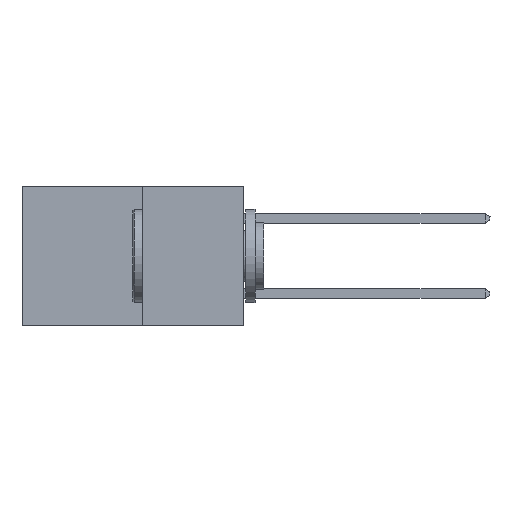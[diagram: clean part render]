
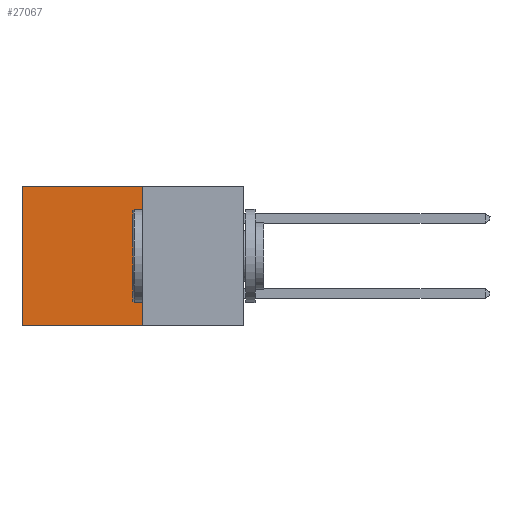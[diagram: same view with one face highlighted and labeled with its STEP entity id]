
A CAD part, left-side view. The second image highlights one B-rep face of the part: STEP entity #27067.
In plain terms, the highlighted planar face has unit normal (-1, 0, 0).
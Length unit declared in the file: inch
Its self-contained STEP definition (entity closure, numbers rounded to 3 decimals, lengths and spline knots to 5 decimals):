
#2558 = EDGE_CURVE ( 'NONE', #7336, #26090, #11444, .T. ) ;
#3672 = CARTESIAN_POINT ( 'NONE',  ( 0.277, 0.27, 0. ) ) ;
#4739 = ORIENTED_EDGE ( 'NONE', *, *, #14288, .F. ) ;
#5889 = PLANE ( 'NONE',  #27256 ) ;
#6470 = VERTEX_POINT ( 'NONE', #24340 ) ;
#7336 = VERTEX_POINT ( 'NONE', #13831 ) ;
#7517 = VERTEX_POINT ( 'NONE', #8390 ) ;
#7743 = ORIENTED_EDGE ( 'NONE', *, *, #2558, .F. ) ;
#7892 = DIRECTION ( 'NONE',  ( 0., 1., 0. ) ) ;
#8390 = CARTESIAN_POINT ( 'NONE',  ( 0.277, 0.59, -0.37 ) ) ;
#8513 = CARTESIAN_POINT ( 'NONE',  ( 0.277, 0.27, -0.37 ) ) ;
#10051 = VECTOR ( 'NONE', #24312, 39.37008 ) ;
#10583 = ORIENTED_EDGE ( 'NONE', *, *, #23178, .T. ) ;
#11107 = DIRECTION ( 'NONE',  ( 0., 0., -1. ) ) ;
#11193 = CARTESIAN_POINT ( 'NONE',  ( 0.277, 0.27, -0.37 ) ) ;
#11444 = LINE ( 'NONE', #11193, #19142 ) ;
#12013 = CARTESIAN_POINT ( 'NONE',  ( 0.277, 0.59, -0.37 ) ) ;
#12015 = ORIENTED_EDGE ( 'NONE', *, *, #32079, .T. ) ;
#12957 = DIRECTION ( 'NONE',  ( 0., 0., -1. ) ) ;
#12999 = CARTESIAN_POINT ( 'NONE',  ( 0.277, 0.27, -0.37 ) ) ;
#13831 = CARTESIAN_POINT ( 'NONE',  ( 0.277, 0.27, 0. ) ) ;
#14288 = EDGE_CURVE ( 'NONE', #26090, #7517, #27508, .T. ) ;
#15849 = VECTOR ( 'NONE', #24981, 39.37008 ) ;
#19142 = VECTOR ( 'NONE', #12957, 39.37008 ) ;
#19477 = CARTESIAN_POINT ( 'NONE',  ( 0.277, 0.27, -0.37 ) ) ;
#20818 = FACE_OUTER_BOUND ( 'NONE', #25191, .T. ) ;
#22686 = LINE ( 'NONE', #12013, #15849 ) ;
#23178 = EDGE_CURVE ( 'NONE', #7336, #6470, #30522, .T. ) ;
#24312 = DIRECTION ( 'NONE',  ( 0., 1., 0. ) ) ;
#24340 = CARTESIAN_POINT ( 'NONE',  ( 0.277, 0.59, 0. ) ) ;
#24981 = DIRECTION ( 'NONE',  ( 0., 0., -1. ) ) ;
#25191 = EDGE_LOOP ( 'NONE', ( #12015, #4739, #7743, #10583 ) ) ;
#26090 = VERTEX_POINT ( 'NONE', #19477 ) ;
#26522 = DIRECTION ( 'NONE',  ( 1., 0., 0. ) ) ;
#26719 = VECTOR ( 'NONE', #7892, 39.37008 ) ;
#27067 = ADVANCED_FACE ( 'NONE', ( #20818 ), #5889, .F. ) ;
#27256 = AXIS2_PLACEMENT_3D ( 'NONE', #8513, #26522, #11107 ) ;
#27508 = LINE ( 'NONE', #12999, #26719 ) ;
#30522 = LINE ( 'NONE', #3672, #10051 ) ;
#32079 = EDGE_CURVE ( 'NONE', #6470, #7517, #22686, .T. ) ;
